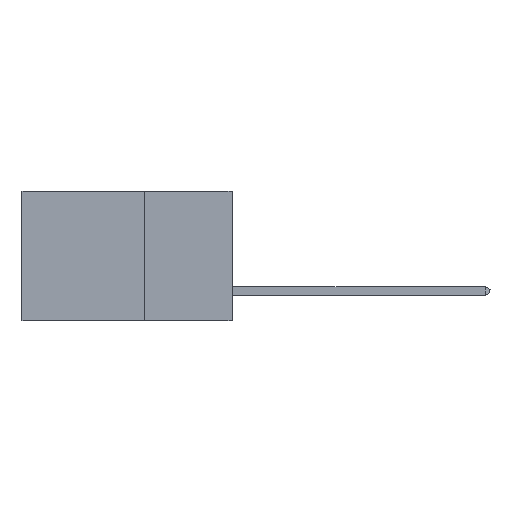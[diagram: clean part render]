
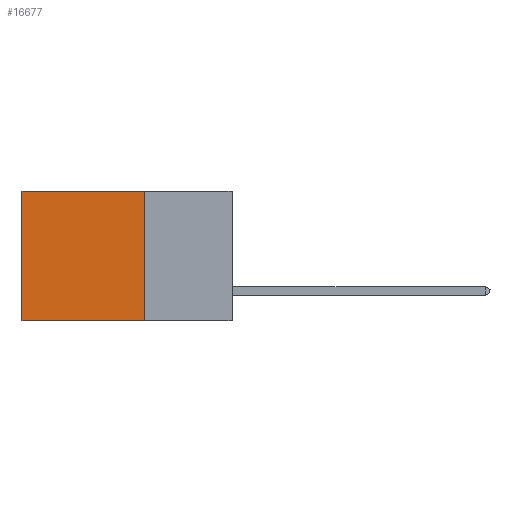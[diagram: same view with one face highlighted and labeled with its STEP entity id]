
A CAD part, left-side view. The second image highlights one B-rep face of the part: STEP entity #16677.
In plain terms, the highlighted planar face has unit normal (-1, 0, 0).
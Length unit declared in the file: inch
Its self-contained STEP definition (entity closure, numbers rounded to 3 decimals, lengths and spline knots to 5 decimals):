
#281 = ORIENTED_EDGE ( 'NONE', *, *, #11355, .F. ) ;
#2239 = ORIENTED_EDGE ( 'NONE', *, *, #20941, .T. ) ;
#2974 = ORIENTED_EDGE ( 'NONE', *, *, #5616, .T. ) ;
#3440 = CARTESIAN_POINT ( 'NONE',  ( 0.2875, 0.25, 0. ) ) ;
#4529 = AXIS2_PLACEMENT_3D ( 'NONE', #20058, #20145, #23997 ) ;
#4728 = DIRECTION ( 'NONE',  ( 0., 1., 0. ) ) ;
#5147 = DIRECTION ( 'NONE',  ( 0., 0., -1. ) ) ;
#5160 = VERTEX_POINT ( 'NONE', #12145 ) ;
#5616 = EDGE_CURVE ( 'NONE', #24313, #5160, #12474, .T. ) ;
#6227 = VECTOR ( 'NONE', #12732, 39.37008 ) ;
#7893 = CARTESIAN_POINT ( 'NONE',  ( 0.2875, 0.25, -0.37 ) ) ;
#7922 = EDGE_LOOP ( 'NONE', ( #2239, #281, #15049, #2974 ) ) ;
#8087 = VECTOR ( 'NONE', #4728, 39.37008 ) ;
#8739 = VECTOR ( 'NONE', #22217, 39.37008 ) ;
#8825 = VECTOR ( 'NONE', #5147, 39.37008 ) ;
#9291 = CARTESIAN_POINT ( 'NONE',  ( 0.2875, 0.6, 0. ) ) ;
#9334 = VERTEX_POINT ( 'NONE', #17259 ) ;
#10045 = VERTEX_POINT ( 'NONE', #17554 ) ;
#10913 = CARTESIAN_POINT ( 'NONE',  ( 0.2875, 0.25, 0. ) ) ;
#11355 = EDGE_CURVE ( 'NONE', #10045, #9334, #18172, .T. ) ;
#12145 = CARTESIAN_POINT ( 'NONE',  ( 0.2875, 0.6, 0. ) ) ;
#12474 = LINE ( 'NONE', #24104, #6227 ) ;
#12732 = DIRECTION ( 'NONE',  ( 0., 1., 0. ) ) ;
#14388 = LINE ( 'NONE', #3440, #8739 ) ;
#15049 = ORIENTED_EDGE ( 'NONE', *, *, #16486, .F. ) ;
#15228 = FACE_OUTER_BOUND ( 'NONE', #7922, .T. ) ;
#16486 = EDGE_CURVE ( 'NONE', #24313, #10045, #14388, .T. ) ;
#16677 = ADVANCED_FACE ( 'NONE', ( #15228 ), #24079, .F. ) ;
#17259 = CARTESIAN_POINT ( 'NONE',  ( 0.2875, 0.6, -0.37 ) ) ;
#17554 = CARTESIAN_POINT ( 'NONE',  ( 0.2875, 0.25, -0.37 ) ) ;
#18172 = LINE ( 'NONE', #7893, #8087 ) ;
#20058 = CARTESIAN_POINT ( 'NONE',  ( 0.2875, 0.25, 0. ) ) ;
#20145 = DIRECTION ( 'NONE',  ( 1., 0., 0. ) ) ;
#20941 = EDGE_CURVE ( 'NONE', #5160, #9334, #24276, .T. ) ;
#22217 = DIRECTION ( 'NONE',  ( 0., 0., -1. ) ) ;
#23997 = DIRECTION ( 'NONE',  ( 0., 0., -1. ) ) ;
#24079 = PLANE ( 'NONE',  #4529 ) ;
#24104 = CARTESIAN_POINT ( 'NONE',  ( 0.2875, 0.25, 0. ) ) ;
#24276 = LINE ( 'NONE', #9291, #8825 ) ;
#24313 = VERTEX_POINT ( 'NONE', #10913 ) ;
